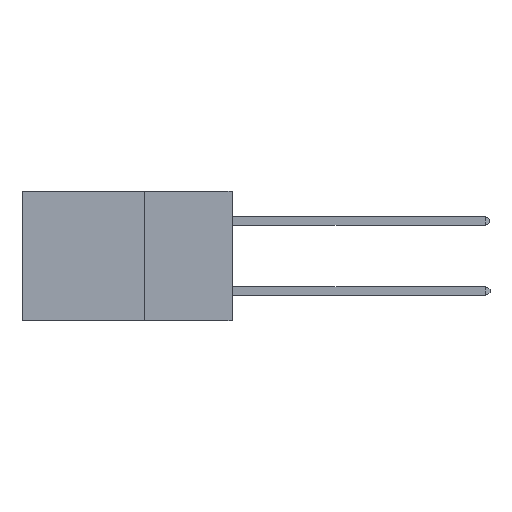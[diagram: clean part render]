
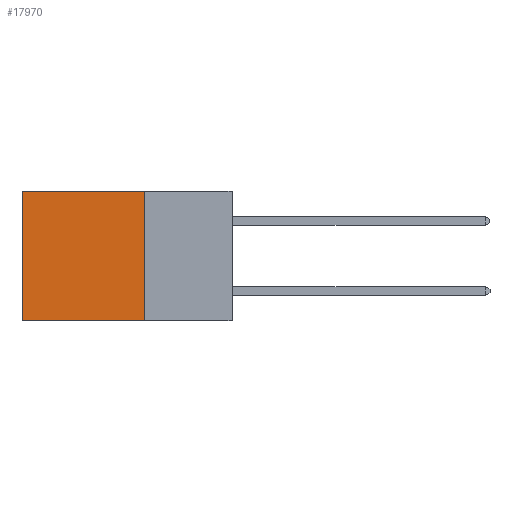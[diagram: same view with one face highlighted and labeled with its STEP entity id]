
A CAD part, left-side view. The second image highlights one B-rep face of the part: STEP entity #17970.
In plain terms, the highlighted planar face has unit normal (-1, 0, 0).
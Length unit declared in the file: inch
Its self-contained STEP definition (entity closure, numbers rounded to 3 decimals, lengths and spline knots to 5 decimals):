
#382 = EDGE_CURVE ( 'NONE', #13283, #9437, #8017, .T. ) ;
#734 = LINE ( 'NONE', #22987, #5404 ) ;
#1759 = DIRECTION ( 'NONE',  ( 0., 0., -1. ) ) ;
#3645 = FACE_OUTER_BOUND ( 'NONE', #10650, .T. ) ;
#4174 = CARTESIAN_POINT ( 'NONE',  ( 0.2875, 0.25, -0.37 ) ) ;
#5042 = AXIS2_PLACEMENT_3D ( 'NONE', #8209, #17649, #6307 ) ;
#5404 = VECTOR ( 'NONE', #1759, 39.37008 ) ;
#6307 = DIRECTION ( 'NONE',  ( 0., 0., -1. ) ) ;
#6964 = ORIENTED_EDGE ( 'NONE', *, *, #13585, .F. ) ;
#7522 = VERTEX_POINT ( 'NONE', #4174 ) ;
#8017 = LINE ( 'NONE', #10443, #12450 ) ;
#8209 = CARTESIAN_POINT ( 'NONE',  ( 0.2875, 0.25, 0. ) ) ;
#8697 = ORIENTED_EDGE ( 'NONE', *, *, #20291, .T. ) ;
#9437 = VERTEX_POINT ( 'NONE', #22329 ) ;
#10443 = CARTESIAN_POINT ( 'NONE',  ( 0.2875, 0.6, 0. ) ) ;
#10650 = EDGE_LOOP ( 'NONE', ( #18655, #17007, #6964, #8697 ) ) ;
#11547 = DIRECTION ( 'NONE',  ( 0., 1., 0. ) ) ;
#12337 = CARTESIAN_POINT ( 'NONE',  ( 0.2875, 0.6, 0. ) ) ;
#12450 = VECTOR ( 'NONE', #13892, 39.37008 ) ;
#13283 = VERTEX_POINT ( 'NONE', #12337 ) ;
#13585 = EDGE_CURVE ( 'NONE', #13710, #7522, #734, .T. ) ;
#13614 = EDGE_CURVE ( 'NONE', #7522, #9437, #19829, .T. ) ;
#13710 = VERTEX_POINT ( 'NONE', #17314 ) ;
#13892 = DIRECTION ( 'NONE',  ( 0., 0., -1. ) ) ;
#14914 = VECTOR ( 'NONE', #15769, 39.37008 ) ;
#15269 = CARTESIAN_POINT ( 'NONE',  ( 0.2875, 0.25, -0.37 ) ) ;
#15769 = DIRECTION ( 'NONE',  ( 0., 1., 0. ) ) ;
#17007 = ORIENTED_EDGE ( 'NONE', *, *, #13614, .F. ) ;
#17314 = CARTESIAN_POINT ( 'NONE',  ( 0.2875, 0.25, 0. ) ) ;
#17503 = LINE ( 'NONE', #24178, #14914 ) ;
#17649 = DIRECTION ( 'NONE',  ( 1., 0., 0. ) ) ;
#17739 = PLANE ( 'NONE',  #5042 ) ;
#17970 = ADVANCED_FACE ( 'NONE', ( #3645 ), #17739, .F. ) ;
#18655 = ORIENTED_EDGE ( 'NONE', *, *, #382, .T. ) ;
#18662 = VECTOR ( 'NONE', #11547, 39.37008 ) ;
#19829 = LINE ( 'NONE', #15269, #18662 ) ;
#20291 = EDGE_CURVE ( 'NONE', #13710, #13283, #17503, .T. ) ;
#22329 = CARTESIAN_POINT ( 'NONE',  ( 0.2875, 0.6, -0.37 ) ) ;
#22987 = CARTESIAN_POINT ( 'NONE',  ( 0.2875, 0.25, 0. ) ) ;
#24178 = CARTESIAN_POINT ( 'NONE',  ( 0.2875, 0.25, 0. ) ) ;
